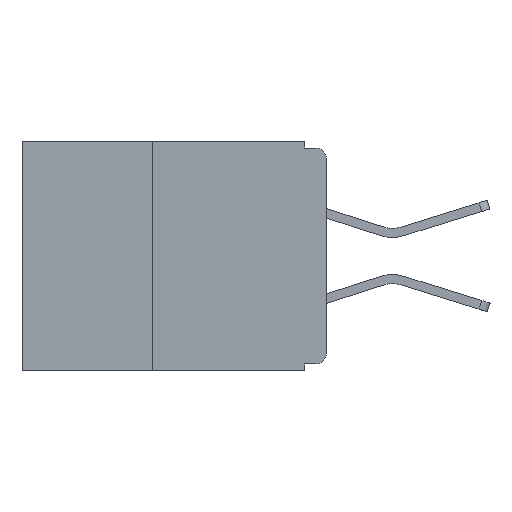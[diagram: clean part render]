
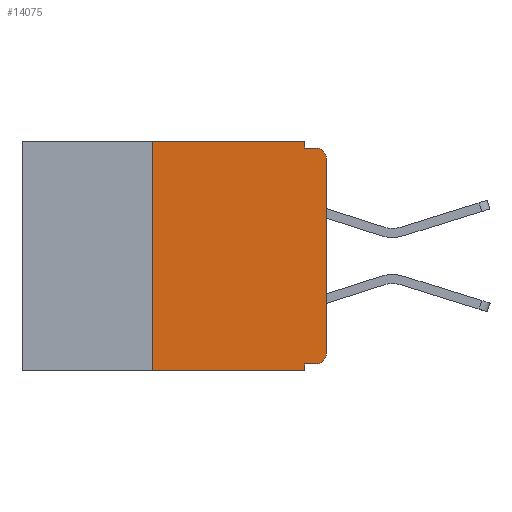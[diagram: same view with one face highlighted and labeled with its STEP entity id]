
A CAD part, left-side view. The second image highlights one B-rep face of the part: STEP entity #14075.
In plain terms, the highlighted planar face has unit normal (-1, 0, 0).
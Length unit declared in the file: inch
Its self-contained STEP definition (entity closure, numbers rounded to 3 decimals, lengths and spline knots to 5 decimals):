
#238 = CARTESIAN_POINT ( 'NONE',  ( 0., 0.031, -0.33 ) ) ;
#431 = LINE ( 'NONE', #3501, #6653 ) ;
#474 = VECTOR ( 'NONE', #7963, 39.37008 ) ;
#603 = VERTEX_POINT ( 'NONE', #8015 ) ;
#757 = DIRECTION ( 'NONE',  ( 0., -1., 0. ) ) ;
#849 = LINE ( 'NONE', #6070, #7436 ) ;
#1016 = EDGE_CURVE ( 'NONE', #14071, #12542, #14372, .T. ) ;
#1290 = CARTESIAN_POINT ( 'NONE',  ( 0., 0., -0.305 ) ) ;
#1387 = EDGE_CURVE ( 'NONE', #12542, #603, #9618, .T. ) ;
#1616 = VERTEX_POINT ( 'NONE', #11539 ) ;
#1862 = CARTESIAN_POINT ( 'NONE',  ( 0., 0.25, 0. ) ) ;
#1892 = AXIS2_PLACEMENT_3D ( 'NONE', #13638, #6103, #14904 ) ;
#2033 = ORIENTED_EDGE ( 'NONE', *, *, #7940, .T. ) ;
#2239 = EDGE_CURVE ( 'NONE', #15319, #4944, #431, .T. ) ;
#2422 = VERTEX_POINT ( 'NONE', #4141 ) ;
#2469 = CARTESIAN_POINT ( 'NONE',  ( 0., 0.031, -0.32 ) ) ;
#2634 = LINE ( 'NONE', #15208, #5737 ) ;
#3501 = CARTESIAN_POINT ( 'NONE',  ( 0., 0.031, -0.33 ) ) ;
#3972 = VERTEX_POINT ( 'NONE', #5488 ) ;
#4022 = LINE ( 'NONE', #7909, #474 ) ;
#4141 = CARTESIAN_POINT ( 'NONE',  ( 0., 0.031, -0.01 ) ) ;
#4404 = DIRECTION ( 'NONE',  ( 0., 0., -1. ) ) ;
#4802 = ORIENTED_EDGE ( 'NONE', *, *, #14631, .F. ) ;
#4944 = VERTEX_POINT ( 'NONE', #238 ) ;
#5488 = CARTESIAN_POINT ( 'NONE',  ( 0., 0.015, -0.01 ) ) ;
#5600 = CARTESIAN_POINT ( 'NONE',  ( 0., 0.25, -0.33 ) ) ;
#5626 = VERTEX_POINT ( 'NONE', #1290 ) ;
#5737 = VECTOR ( 'NONE', #16161, 39.37008 ) ;
#5767 = EDGE_CURVE ( 'NONE', #2422, #3972, #2634, .T. ) ;
#5834 = ORIENTED_EDGE ( 'NONE', *, *, #10313, .T. ) ;
#6070 = CARTESIAN_POINT ( 'NONE',  ( 0., 0.437, -0.33 ) ) ;
#6103 = DIRECTION ( 'NONE',  ( -1., 0., 0. ) ) ;
#6132 = ORIENTED_EDGE ( 'NONE', *, *, #11068, .T. ) ;
#6179 = ORIENTED_EDGE ( 'NONE', *, *, #1016, .F. ) ;
#6276 = VECTOR ( 'NONE', #757, 39.37008 ) ;
#6502 = CARTESIAN_POINT ( 'NONE',  ( 0., 0.25, -0.33 ) ) ;
#6553 = DIRECTION ( 'NONE',  ( 1., 0., 0. ) ) ;
#6653 = VECTOR ( 'NONE', #4404, 39.37008 ) ;
#6723 = VECTOR ( 'NONE', #16400, 39.37008 ) ;
#6965 = EDGE_CURVE ( 'NONE', #9578, #5626, #15723, .T. ) ;
#7312 = AXIS2_PLACEMENT_3D ( 'NONE', #14078, #6553, #15343 ) ;
#7349 = EDGE_LOOP ( 'NONE', ( #6132, #5834, #15685, #4802, #10698, #6179, #2033, #12110, #15459, #8689 ) ) ;
#7436 = VECTOR ( 'NONE', #12356, 39.37008 ) ;
#7746 = VECTOR ( 'NONE', #13982, 39.37008 ) ;
#7748 = CARTESIAN_POINT ( 'NONE',  ( 0., 0., 0. ) ) ;
#7909 = CARTESIAN_POINT ( 'NONE',  ( 0., 0., -0.32 ) ) ;
#7940 = EDGE_CURVE ( 'NONE', #14071, #4944, #849, .T. ) ;
#7963 = DIRECTION ( 'NONE',  ( 0., 1., 0. ) ) ;
#8015 = CARTESIAN_POINT ( 'NONE',  ( 0., 0.031, 0. ) ) ;
#8488 = DIRECTION ( 'NONE',  ( 0., 0., -1. ) ) ;
#8489 = VECTOR ( 'NONE', #15515, 39.37008 ) ;
#8525 = DIRECTION ( 'NONE',  ( -1., 0., 0. ) ) ;
#8542 = CARTESIAN_POINT ( 'NONE',  ( 0., 0.015, -0.305 ) ) ;
#8689 = ORIENTED_EDGE ( 'NONE', *, *, #6965, .T. ) ;
#8730 = FACE_OUTER_BOUND ( 'NONE', #7349, .T. ) ;
#9578 = VERTEX_POINT ( 'NONE', #14761 ) ;
#9618 = LINE ( 'NONE', #10240, #6276 ) ;
#10240 = CARTESIAN_POINT ( 'NONE',  ( 0., 0.437, 0. ) ) ;
#10287 = PLANE ( 'NONE',  #7312 ) ;
#10313 = EDGE_CURVE ( 'NONE', #1616, #3972, #16186, .T. ) ;
#10698 = ORIENTED_EDGE ( 'NONE', *, *, #1387, .F. ) ;
#11068 = EDGE_CURVE ( 'NONE', #5626, #1616, #14430, .T. ) ;
#11539 = CARTESIAN_POINT ( 'NONE',  ( 0., 0., -0.025 ) ) ;
#11780 = AXIS2_PLACEMENT_3D ( 'NONE', #8542, #8525, #8488 ) ;
#12110 = ORIENTED_EDGE ( 'NONE', *, *, #2239, .F. ) ;
#12356 = DIRECTION ( 'NONE',  ( 0., -1., 0. ) ) ;
#12542 = VERTEX_POINT ( 'NONE', #1862 ) ;
#13638 = CARTESIAN_POINT ( 'NONE',  ( 0., 0.015, -0.025 ) ) ;
#13792 = LINE ( 'NONE', #15161, #6723 ) ;
#13982 = DIRECTION ( 'NONE',  ( 0., 0., 1. ) ) ;
#14071 = VERTEX_POINT ( 'NONE', #6502 ) ;
#14075 = ADVANCED_FACE ( 'NONE', ( #8730 ), #10287, .F. ) ;
#14078 = CARTESIAN_POINT ( 'NONE',  ( 0., 0.437, 0. ) ) ;
#14372 = LINE ( 'NONE', #5600, #8489 ) ;
#14430 = LINE ( 'NONE', #7748, #7746 ) ;
#14631 = EDGE_CURVE ( 'NONE', #603, #2422, #13792, .T. ) ;
#14761 = CARTESIAN_POINT ( 'NONE',  ( 0., 0.015, -0.32 ) ) ;
#14904 = DIRECTION ( 'NONE',  ( 0., 0., -1. ) ) ;
#15161 = CARTESIAN_POINT ( 'NONE',  ( 0., 0.031, 0. ) ) ;
#15208 = CARTESIAN_POINT ( 'NONE',  ( 0., 0., -0.01 ) ) ;
#15319 = VERTEX_POINT ( 'NONE', #2469 ) ;
#15343 = DIRECTION ( 'NONE',  ( 0., 0., -1. ) ) ;
#15450 = EDGE_CURVE ( 'NONE', #9578, #15319, #4022, .T. ) ;
#15459 = ORIENTED_EDGE ( 'NONE', *, *, #15450, .F. ) ;
#15515 = DIRECTION ( 'NONE',  ( 0., 0., 1. ) ) ;
#15685 = ORIENTED_EDGE ( 'NONE', *, *, #5767, .F. ) ;
#15723 = CIRCLE ( 'NONE', #11780, 0.015 ) ;
#16161 = DIRECTION ( 'NONE',  ( 0., -1., 0. ) ) ;
#16186 = CIRCLE ( 'NONE', #1892, 0.015 ) ;
#16400 = DIRECTION ( 'NONE',  ( 0., 0., -1. ) ) ;
